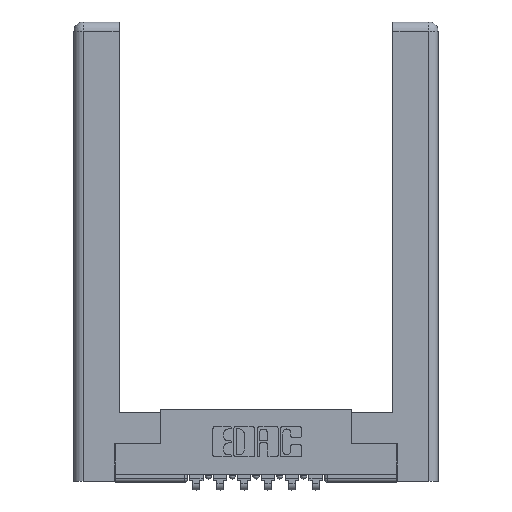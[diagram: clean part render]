
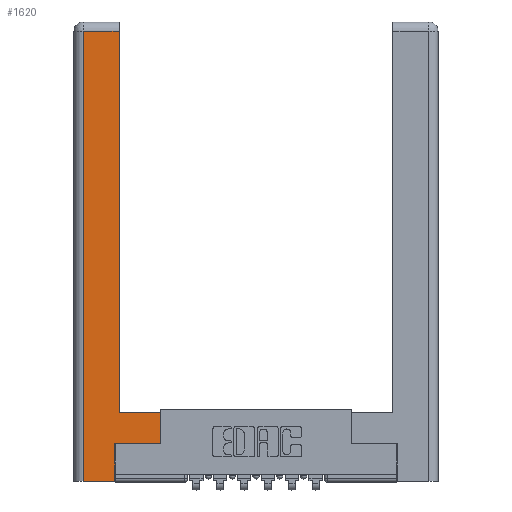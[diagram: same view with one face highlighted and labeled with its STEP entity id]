
A CAD part, top view. The second image highlights one B-rep face of the part: STEP entity #1620.
In plain terms, the highlighted planar face has unit normal (0, 0, 1).
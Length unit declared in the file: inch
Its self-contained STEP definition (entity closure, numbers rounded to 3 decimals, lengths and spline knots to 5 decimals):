
#126 = ORIENTED_EDGE ( 'NONE', *, *, #2186, .T. ) ;
#143 = ORIENTED_EDGE ( 'NONE', *, *, #8241, .T. ) ;
#984 = VECTOR ( 'NONE', #5677, 39.37008 ) ;
#988 = VERTEX_POINT ( 'NONE', #2566 ) ;
#1212 = CARTESIAN_POINT ( 'NONE',  ( 0.295, 0.45, 0. ) ) ;
#1418 = VERTEX_POINT ( 'NONE', #3989 ) ;
#1565 = VECTOR ( 'NONE', #2072, 39.37008 ) ;
#1620 = ADVANCED_FACE ( 'NONE', ( #2409 ), #12325, .F. ) ;
#1655 = LINE ( 'NONE', #12503, #984 ) ;
#1738 = EDGE_CURVE ( 'NONE', #3113, #2882, #7686, .T. ) ;
#2062 = CARTESIAN_POINT ( 'NONE',  ( 0.565, 0.245, 0. ) ) ;
#2072 = DIRECTION ( 'NONE',  ( -1., 0., 0. ) ) ;
#2113 = LINE ( 'NONE', #11301, #2552 ) ;
#2186 = EDGE_CURVE ( 'NONE', #2720, #6006, #1655, .T. ) ;
#2256 = ORIENTED_EDGE ( 'NONE', *, *, #5325, .T. ) ;
#2285 = CARTESIAN_POINT ( 'NONE',  ( 0.265, 0.245, 0. ) ) ;
#2409 = FACE_OUTER_BOUND ( 'NONE', #5573, .T. ) ;
#2552 = VECTOR ( 'NONE', #6143, 39.37008 ) ;
#2566 = CARTESIAN_POINT ( 'NONE',  ( 0.295, 0.45, 0. ) ) ;
#2663 = DIRECTION ( 'NONE',  ( 0., 1., 0. ) ) ;
#2720 = VERTEX_POINT ( 'NONE', #10926 ) ;
#2882 = VERTEX_POINT ( 'NONE', #7430 ) ;
#2970 = EDGE_CURVE ( 'NONE', #6006, #6998, #4712, .T. ) ;
#3004 = VERTEX_POINT ( 'NONE', #11524 ) ;
#3113 = VERTEX_POINT ( 'NONE', #2062 ) ;
#3989 = CARTESIAN_POINT ( 'NONE',  ( 0.265, 0.245, 0. ) ) ;
#4114 = CARTESIAN_POINT ( 'NONE',  ( 0.0615, 0., 0. ) ) ;
#4215 = CARTESIAN_POINT ( 'NONE',  ( 0.295, 3., 0. ) ) ;
#4712 = LINE ( 'NONE', #9794, #9657 ) ;
#5190 = LINE ( 'NONE', #4215, #12068 ) ;
#5300 = DIRECTION ( 'NONE',  ( 0., 0., -1. ) ) ;
#5325 = EDGE_CURVE ( 'NONE', #3004, #2720, #9763, .T. ) ;
#5467 = ORIENTED_EDGE ( 'NONE', *, *, #10623, .T. ) ;
#5573 = EDGE_LOOP ( 'NONE', ( #143, #2256, #126, #11848, #5467, #6722, #8982, #8020 ) ) ;
#5677 = DIRECTION ( 'NONE',  ( 0., -1., 0. ) ) ;
#6006 = VERTEX_POINT ( 'NONE', #4114 ) ;
#6143 = DIRECTION ( 'NONE',  ( 1., 0., 0. ) ) ;
#6202 = VECTOR ( 'NONE', #8420, 39.37008 ) ;
#6502 = AXIS2_PLACEMENT_3D ( 'NONE', #8340, #5300, #11261 ) ;
#6722 = ORIENTED_EDGE ( 'NONE', *, *, #7787, .T. ) ;
#6865 = DIRECTION ( 'NONE',  ( -1., 0., 0. ) ) ;
#6998 = VERTEX_POINT ( 'NONE', #8359 ) ;
#7430 = CARTESIAN_POINT ( 'NONE',  ( 0.565, 0.45, 0. ) ) ;
#7686 = LINE ( 'NONE', #11721, #12779 ) ;
#7787 = EDGE_CURVE ( 'NONE', #1418, #3113, #2113, .T. ) ;
#8020 = ORIENTED_EDGE ( 'NONE', *, *, #12249, .T. ) ;
#8241 = EDGE_CURVE ( 'NONE', #988, #3004, #5190, .T. ) ;
#8340 = CARTESIAN_POINT ( 'NONE',  ( 0., 0., 0. ) ) ;
#8359 = CARTESIAN_POINT ( 'NONE',  ( 0.265, 0., 0. ) ) ;
#8420 = DIRECTION ( 'NONE',  ( 0., 1., 0. ) ) ;
#8775 = CARTESIAN_POINT ( 'NONE',  ( 0.0615, 2.94, 0. ) ) ;
#8819 = VECTOR ( 'NONE', #6865, 39.37008 ) ;
#8982 = ORIENTED_EDGE ( 'NONE', *, *, #1738, .T. ) ;
#9657 = VECTOR ( 'NONE', #12709, 39.37008 ) ;
#9763 = LINE ( 'NONE', #8775, #8819 ) ;
#9794 = CARTESIAN_POINT ( 'NONE',  ( 0.265, 0., 0. ) ) ;
#10285 = DIRECTION ( 'NONE',  ( 0., 1., 0. ) ) ;
#10623 = EDGE_CURVE ( 'NONE', #6998, #1418, #11340, .T. ) ;
#10926 = CARTESIAN_POINT ( 'NONE',  ( 0.0615, 2.94, 0. ) ) ;
#11261 = DIRECTION ( 'NONE',  ( -1., 0., 0. ) ) ;
#11301 = CARTESIAN_POINT ( 'NONE',  ( 0.565, 0.245, 0. ) ) ;
#11340 = LINE ( 'NONE', #2285, #6202 ) ;
#11524 = CARTESIAN_POINT ( 'NONE',  ( 0.295, 2.94, 0. ) ) ;
#11721 = CARTESIAN_POINT ( 'NONE',  ( 0.565, 0.45, 0. ) ) ;
#11848 = ORIENTED_EDGE ( 'NONE', *, *, #2970, .T. ) ;
#12068 = VECTOR ( 'NONE', #10285, 39.37008 ) ;
#12249 = EDGE_CURVE ( 'NONE', #2882, #988, #12393, .T. ) ;
#12325 = PLANE ( 'NONE',  #6502 ) ;
#12393 = LINE ( 'NONE', #1212, #1565 ) ;
#12503 = CARTESIAN_POINT ( 'NONE',  ( 0.0615, 0., 0. ) ) ;
#12709 = DIRECTION ( 'NONE',  ( 1., 0., 0. ) ) ;
#12779 = VECTOR ( 'NONE', #2663, 39.37008 ) ;
